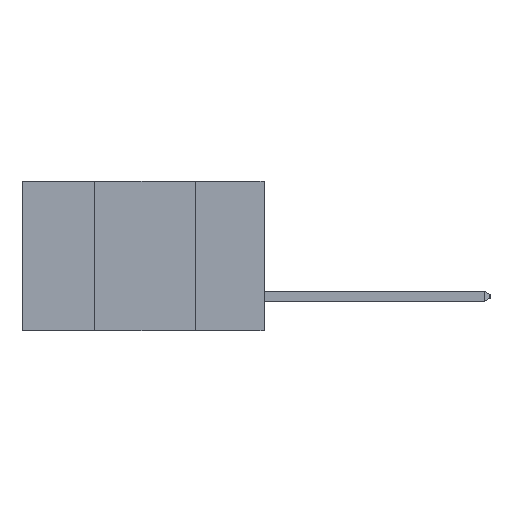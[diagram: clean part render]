
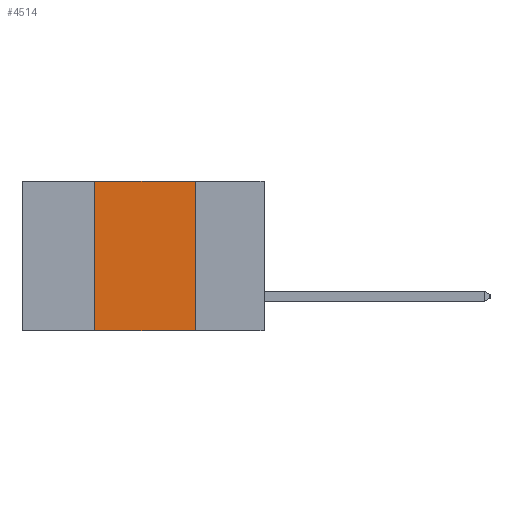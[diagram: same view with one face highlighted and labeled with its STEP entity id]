
A CAD part, left-side view. The second image highlights one B-rep face of the part: STEP entity #4514.
In plain terms, the highlighted planar face has unit normal (-1, 0, 0).
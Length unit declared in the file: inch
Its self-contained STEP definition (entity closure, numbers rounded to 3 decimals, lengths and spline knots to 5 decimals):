
#225 = EDGE_CURVE ( 'NONE', #1098, #16941, #7780, .T. ) ;
#965 = CARTESIAN_POINT ( 'NONE',  ( 0., 0.42, 0. ) ) ;
#1098 = VERTEX_POINT ( 'NONE', #965 ) ;
#2148 = DIRECTION ( 'NONE',  ( 0., 0., -1. ) ) ;
#2151 = DIRECTION ( 'NONE',  ( 1., 0., 0. ) ) ;
#2189 = CARTESIAN_POINT ( 'NONE',  ( 0., 0.6, 0. ) ) ;
#2211 = EDGE_CURVE ( 'NONE', #16941, #8614, #12829, .T. ) ;
#2214 = ORIENTED_EDGE ( 'NONE', *, *, #17503, .F. ) ;
#2250 = VECTOR ( 'NONE', #12623, 39.37008 ) ;
#2627 = PLANE ( 'NONE',  #3287 ) ;
#3091 = DIRECTION ( 'NONE',  ( 0., 0., -1. ) ) ;
#3287 = AXIS2_PLACEMENT_3D ( 'NONE', #2189, #2151, #2148 ) ;
#3496 = DIRECTION ( 'NONE',  ( 0., -1., 0. ) ) ;
#3618 = ORIENTED_EDGE ( 'NONE', *, *, #225, .F. ) ;
#3757 = VECTOR ( 'NONE', #15426, 39.37008 ) ;
#3777 = ORIENTED_EDGE ( 'NONE', *, *, #2211, .F. ) ;
#4386 = VECTOR ( 'NONE', #3091, 39.37008 ) ;
#4514 = ADVANCED_FACE ( 'NONE', ( #15851 ), #2627, .F. ) ;
#4939 = CARTESIAN_POINT ( 'NONE',  ( 0., 0.6, -0.37 ) ) ;
#5086 = CARTESIAN_POINT ( 'NONE',  ( 0., 0.42, -0.37 ) ) ;
#5578 = LINE ( 'NONE', #4939, #13108 ) ;
#6097 = VERTEX_POINT ( 'NONE', #13371 ) ;
#6534 = CARTESIAN_POINT ( 'NONE',  ( 0., 0.17, 0. ) ) ;
#7780 = LINE ( 'NONE', #16729, #3757 ) ;
#8614 = VERTEX_POINT ( 'NONE', #19096 ) ;
#10177 = LINE ( 'NONE', #5086, #2250 ) ;
#10814 = ORIENTED_EDGE ( 'NONE', *, *, #14608, .T. ) ;
#12623 = DIRECTION ( 'NONE',  ( 0., 0., 1. ) ) ;
#12829 = LINE ( 'NONE', #16782, #4386 ) ;
#13108 = VECTOR ( 'NONE', #3496, 39.37008 ) ;
#13201 = EDGE_LOOP ( 'NONE', ( #3777, #3618, #2214, #10814 ) ) ;
#13371 = CARTESIAN_POINT ( 'NONE',  ( 0., 0.42, -0.37 ) ) ;
#14608 = EDGE_CURVE ( 'NONE', #6097, #8614, #5578, .T. ) ;
#15426 = DIRECTION ( 'NONE',  ( 0., -1., 0. ) ) ;
#15851 = FACE_OUTER_BOUND ( 'NONE', #13201, .T. ) ;
#16729 = CARTESIAN_POINT ( 'NONE',  ( 0., 0.6, 0. ) ) ;
#16782 = CARTESIAN_POINT ( 'NONE',  ( 0., 0.17, -0.37 ) ) ;
#16941 = VERTEX_POINT ( 'NONE', #6534 ) ;
#17503 = EDGE_CURVE ( 'NONE', #6097, #1098, #10177, .T. ) ;
#19096 = CARTESIAN_POINT ( 'NONE',  ( 0., 0.17, -0.37 ) ) ;
